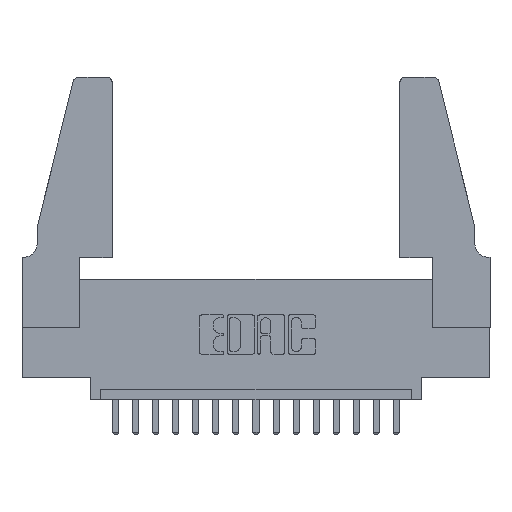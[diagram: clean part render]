
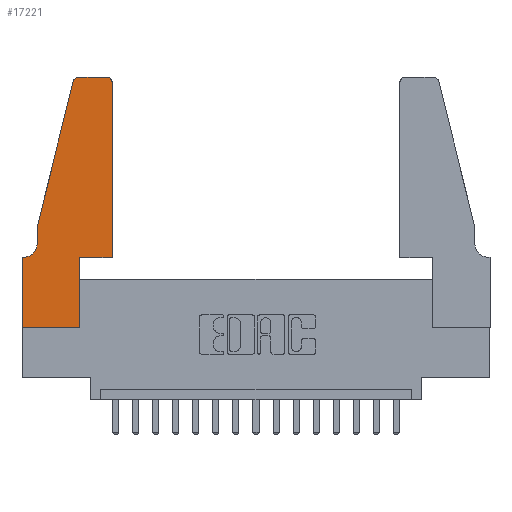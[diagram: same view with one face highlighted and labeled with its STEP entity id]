
A CAD part, top view. The second image highlights one B-rep face of the part: STEP entity #17221.
In plain terms, the highlighted planar face has unit normal (0, 0, 1).
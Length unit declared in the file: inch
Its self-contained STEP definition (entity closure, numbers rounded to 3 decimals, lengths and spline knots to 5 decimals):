
#189 = DIRECTION ( 'NONE',  ( -0.239, -0.971, 0. ) ) ;
#300 = DIRECTION ( 'NONE',  ( -1., 0., 0. ) ) ;
#323 = LINE ( 'NONE', #12463, #940 ) ;
#635 = VERTEX_POINT ( 'NONE', #2222 ) ;
#921 = CARTESIAN_POINT ( 'NONE',  ( 0.0755, 0.42, 0.37 ) ) ;
#940 = VECTOR ( 'NONE', #14834, 39.37008 ) ;
#970 = ORIENTED_EDGE ( 'NONE', *, *, #15128, .T. ) ;
#1103 = VERTEX_POINT ( 'NONE', #3077 ) ;
#1194 = VECTOR ( 'NONE', #15991, 39.37008 ) ;
#1633 = ORIENTED_EDGE ( 'NONE', *, *, #11261, .T. ) ;
#1691 = VERTEX_POINT ( 'NONE', #11052 ) ;
#2047 = EDGE_CURVE ( 'NONE', #10865, #13839, #7677, .T. ) ;
#2053 = VERTEX_POINT ( 'NONE', #9687 ) ;
#2123 = AXIS2_PLACEMENT_3D ( 'NONE', #17128, #2443, #6448 ) ;
#2222 = CARTESIAN_POINT ( 'NONE',  ( 0.0055, 0.35, 0.37 ) ) ;
#2443 = DIRECTION ( 'NONE',  ( 0., 0., -1. ) ) ;
#2463 = LINE ( 'NONE', #12030, #16900 ) ;
#3077 = CARTESIAN_POINT ( 'NONE',  ( 0.2865, 0., 0.37 ) ) ;
#3194 = ORIENTED_EDGE ( 'NONE', *, *, #9220, .T. ) ;
#3734 = VECTOR ( 'NONE', #10701, 39.37008 ) ;
#3879 = LINE ( 'NONE', #9891, #4526 ) ;
#4092 = LINE ( 'NONE', #10224, #5966 ) ;
#4213 = LINE ( 'NONE', #6846, #15429 ) ;
#4223 = DIRECTION ( 'NONE',  ( 0., 1., 0. ) ) ;
#4499 = LINE ( 'NONE', #4531, #12413 ) ;
#4526 = VECTOR ( 'NONE', #8339, 39.37008 ) ;
#4531 = CARTESIAN_POINT ( 'NONE',  ( 0.0755, 0.35, 0.37 ) ) ;
#4940 = DIRECTION ( 'NONE',  ( 1., 0., 0. ) ) ;
#4973 = ORIENTED_EDGE ( 'NONE', *, *, #8229, .T. ) ;
#5475 = CIRCLE ( 'NONE', #2123, 0.07 ) ;
#5498 = CARTESIAN_POINT ( 'NONE',  ( 0., 0., 0.37 ) ) ;
#5696 = ORIENTED_EDGE ( 'NONE', *, *, #16543, .T. ) ;
#5783 = EDGE_CURVE ( 'NONE', #1103, #7719, #4213, .T. ) ;
#5966 = VECTOR ( 'NONE', #12810, 39.37008 ) ;
#6031 = LINE ( 'NONE', #5498, #3734 ) ;
#6370 = ORIENTED_EDGE ( 'NONE', *, *, #14004, .T. ) ;
#6448 = DIRECTION ( 'NONE',  ( -1., 0., 0. ) ) ;
#6815 = CARTESIAN_POINT ( 'NONE',  ( 0.0755, 0.5, 0.37 ) ) ;
#6846 = CARTESIAN_POINT ( 'NONE',  ( 0.2865, 0.35, 0.37 ) ) ;
#6878 = ORIENTED_EDGE ( 'NONE', *, *, #5783, .T. ) ;
#6886 = CIRCLE ( 'NONE', #13566, 0.03 ) ;
#7019 = LINE ( 'NONE', #6815, #8882 ) ;
#7191 = AXIS2_PLACEMENT_3D ( 'NONE', #8563, #11529, #4940 ) ;
#7243 = DIRECTION ( 'NONE',  ( 0., 0., 1. ) ) ;
#7677 = CIRCLE ( 'NONE', #7191, 0.03 ) ;
#7719 = VERTEX_POINT ( 'NONE', #12741 ) ;
#7805 = CARTESIAN_POINT ( 'NONE',  ( 0.284, 1.22, 0.37 ) ) ;
#8229 = EDGE_CURVE ( 'NONE', #10703, #635, #5475, .T. ) ;
#8246 = VERTEX_POINT ( 'NONE', #9371 ) ;
#8339 = DIRECTION ( 'NONE',  ( 0., -1., 0. ) ) ;
#8370 = DIRECTION ( 'NONE',  ( 1., 0., 0. ) ) ;
#8563 = CARTESIAN_POINT ( 'NONE',  ( 0.4205, 1.22, 0.37 ) ) ;
#8882 = VECTOR ( 'NONE', #189, 39.37008 ) ;
#9220 = EDGE_CURVE ( 'NONE', #14825, #2053, #6886, .T. ) ;
#9358 = LINE ( 'NONE', #9373, #1194 ) ;
#9371 = CARTESIAN_POINT ( 'NONE',  ( 0., 0., 0.37 ) ) ;
#9373 = CARTESIAN_POINT ( 'NONE',  ( 0.4505, 0.35, 0.37 ) ) ;
#9578 = VERTEX_POINT ( 'NONE', #13040 ) ;
#9687 = CARTESIAN_POINT ( 'NONE',  ( 0.25487, 1.22718, 0.37 ) ) ;
#9815 = CARTESIAN_POINT ( 'NONE',  ( 0.0755, 0.5, 0.37 ) ) ;
#9891 = CARTESIAN_POINT ( 'NONE',  ( 0.0755, 0.5, 0.37 ) ) ;
#10155 = ORIENTED_EDGE ( 'NONE', *, *, #11242, .T. ) ;
#10224 = CARTESIAN_POINT ( 'NONE',  ( 0., 0., 0.37 ) ) ;
#10701 = DIRECTION ( 'NONE',  ( 1., 0., 0. ) ) ;
#10703 = VERTEX_POINT ( 'NONE', #921 ) ;
#10865 = VERTEX_POINT ( 'NONE', #15196 ) ;
#11052 = CARTESIAN_POINT ( 'NONE',  ( 0., 0.35, 0.37 ) ) ;
#11242 = EDGE_CURVE ( 'NONE', #17298, #10703, #3879, .T. ) ;
#11261 = EDGE_CURVE ( 'NONE', #13839, #14825, #323, .T. ) ;
#11529 = DIRECTION ( 'NONE',  ( 0., 0., 1. ) ) ;
#12030 = CARTESIAN_POINT ( 'NONE',  ( 0.4505, 0.35, 0.37 ) ) ;
#12037 = DIRECTION ( 'NONE',  ( 0., 0., 1. ) ) ;
#12372 = PLANE ( 'NONE',  #13538 ) ;
#12413 = VECTOR ( 'NONE', #300, 39.37008 ) ;
#12463 = CARTESIAN_POINT ( 'NONE',  ( 0.2605, 1.25, 0.37 ) ) ;
#12670 = ORIENTED_EDGE ( 'NONE', *, *, #2047, .T. ) ;
#12673 = ORIENTED_EDGE ( 'NONE', *, *, #14515, .T. ) ;
#12741 = CARTESIAN_POINT ( 'NONE',  ( 0.2865, 0.35, 0.37 ) ) ;
#12810 = DIRECTION ( 'NONE',  ( 0., -1., 0. ) ) ;
#13040 = CARTESIAN_POINT ( 'NONE',  ( 0.4505, 0.35, 0.37 ) ) ;
#13260 = ORIENTED_EDGE ( 'NONE', *, *, #16492, .T. ) ;
#13538 = AXIS2_PLACEMENT_3D ( 'NONE', #15203, #7243, #8370 ) ;
#13566 = AXIS2_PLACEMENT_3D ( 'NONE', #7805, #12037, #13941 ) ;
#13618 = FACE_OUTER_BOUND ( 'NONE', #15750, .T. ) ;
#13839 = VERTEX_POINT ( 'NONE', #16968 ) ;
#13941 = DIRECTION ( 'NONE',  ( 1., 0., 0. ) ) ;
#14004 = EDGE_CURVE ( 'NONE', #7719, #9578, #2463, .T. ) ;
#14515 = EDGE_CURVE ( 'NONE', #8246, #1103, #6031, .T. ) ;
#14825 = VERTEX_POINT ( 'NONE', #15462 ) ;
#14834 = DIRECTION ( 'NONE',  ( -1., 0., 0. ) ) ;
#15005 = ORIENTED_EDGE ( 'NONE', *, *, #16171, .T. ) ;
#15128 = EDGE_CURVE ( 'NONE', #9578, #10865, #9358, .T. ) ;
#15196 = CARTESIAN_POINT ( 'NONE',  ( 0.4505, 1.22, 0.37 ) ) ;
#15203 = CARTESIAN_POINT ( 'NONE',  ( 0., 0.35, 0.37 ) ) ;
#15429 = VECTOR ( 'NONE', #4223, 39.37008 ) ;
#15462 = CARTESIAN_POINT ( 'NONE',  ( 0.284, 1.25, 0.37 ) ) ;
#15750 = EDGE_LOOP ( 'NONE', ( #1633, #3194, #13260, #10155, #4973, #5696, #15005, #12673, #6878, #6370, #970, #12670 ) ) ;
#15991 = DIRECTION ( 'NONE',  ( 0., 1., 0. ) ) ;
#16171 = EDGE_CURVE ( 'NONE', #1691, #8246, #4092, .T. ) ;
#16174 = DIRECTION ( 'NONE',  ( 1., 0., 0. ) ) ;
#16492 = EDGE_CURVE ( 'NONE', #2053, #17298, #7019, .T. ) ;
#16543 = EDGE_CURVE ( 'NONE', #635, #1691, #4499, .T. ) ;
#16900 = VECTOR ( 'NONE', #16174, 39.37008 ) ;
#16968 = CARTESIAN_POINT ( 'NONE',  ( 0.4205, 1.25, 0.37 ) ) ;
#17128 = CARTESIAN_POINT ( 'NONE',  ( 0.0055, 0.42, 0.37 ) ) ;
#17221 = ADVANCED_FACE ( 'NONE', ( #13618 ), #12372, .T. ) ;
#17298 = VERTEX_POINT ( 'NONE', #9815 ) ;
